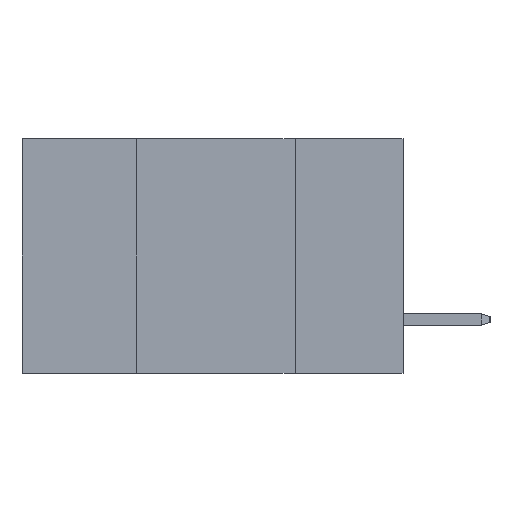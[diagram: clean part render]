
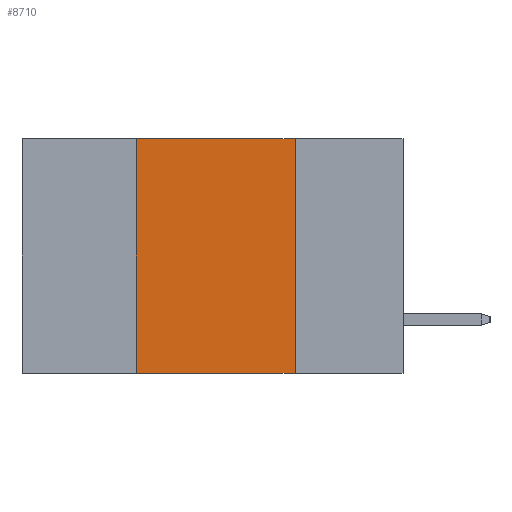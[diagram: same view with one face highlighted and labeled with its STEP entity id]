
A CAD part, left-side view. The second image highlights one B-rep face of the part: STEP entity #8710.
In plain terms, the highlighted planar face has unit normal (-1, 0, 0).
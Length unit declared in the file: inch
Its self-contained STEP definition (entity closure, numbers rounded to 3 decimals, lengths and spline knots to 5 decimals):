
#149 = CARTESIAN_POINT ( 'NONE',  ( 0., 0.6, 0. ) ) ;
#259 = CARTESIAN_POINT ( 'NONE',  ( 0., 0.6, -0.37 ) ) ;
#408 = EDGE_CURVE ( 'NONE', #11132, #8319, #11571, .T. ) ;
#747 = DIRECTION ( 'NONE',  ( 0., -1., 0. ) ) ;
#798 = CARTESIAN_POINT ( 'NONE',  ( 0., 0.42, 0. ) ) ;
#871 = CARTESIAN_POINT ( 'NONE',  ( 0., 0.42, 0. ) ) ;
#2020 = DIRECTION ( 'NONE',  ( 0., 0., -1. ) ) ;
#2052 = DIRECTION ( 'NONE',  ( 0., 0., -1. ) ) ;
#2926 = CARTESIAN_POINT ( 'NONE',  ( 0., 0.17, -0.37 ) ) ;
#3277 = EDGE_LOOP ( 'NONE', ( #5813, #7336, #9105, #10205 ) ) ;
#3893 = LINE ( 'NONE', #259, #6085 ) ;
#4747 = FACE_OUTER_BOUND ( 'NONE', #3277, .T. ) ;
#5245 = VECTOR ( 'NONE', #747, 39.37008 ) ;
#5610 = CARTESIAN_POINT ( 'NONE',  ( 0., 0.17, 0. ) ) ;
#5813 = ORIENTED_EDGE ( 'NONE', *, *, #9576, .F. ) ;
#6085 = VECTOR ( 'NONE', #10546, 39.37008 ) ;
#7280 = VECTOR ( 'NONE', #2052, 39.37008 ) ;
#7332 = CARTESIAN_POINT ( 'NONE',  ( 0., 0.42, -0.37 ) ) ;
#7336 = ORIENTED_EDGE ( 'NONE', *, *, #408, .F. ) ;
#8319 = VERTEX_POINT ( 'NONE', #9037 ) ;
#8391 = LINE ( 'NONE', #5610, #7280 ) ;
#8603 = PLANE ( 'NONE',  #8829 ) ;
#8710 = ADVANCED_FACE ( 'NONE', ( #4747 ), #8603, .F. ) ;
#8829 = AXIS2_PLACEMENT_3D ( 'NONE', #149, #11296, #2020 ) ;
#9037 = CARTESIAN_POINT ( 'NONE',  ( 0., 0.17, 0. ) ) ;
#9105 = ORIENTED_EDGE ( 'NONE', *, *, #11438, .F. ) ;
#9576 = EDGE_CURVE ( 'NONE', #8319, #11983, #8391, .T. ) ;
#9698 = CARTESIAN_POINT ( 'NONE',  ( 0., 0.6, 0. ) ) ;
#9874 = VERTEX_POINT ( 'NONE', #7332 ) ;
#10132 = DIRECTION ( 'NONE',  ( 0., 0., 1. ) ) ;
#10205 = ORIENTED_EDGE ( 'NONE', *, *, #10398, .T. ) ;
#10398 = EDGE_CURVE ( 'NONE', #9874, #11983, #3893, .T. ) ;
#10546 = DIRECTION ( 'NONE',  ( 0., -1., 0. ) ) ;
#10855 = LINE ( 'NONE', #798, #11397 ) ;
#11132 = VERTEX_POINT ( 'NONE', #871 ) ;
#11296 = DIRECTION ( 'NONE',  ( 1., 0., 0. ) ) ;
#11397 = VECTOR ( 'NONE', #10132, 39.37008 ) ;
#11438 = EDGE_CURVE ( 'NONE', #9874, #11132, #10855, .T. ) ;
#11571 = LINE ( 'NONE', #9698, #5245 ) ;
#11983 = VERTEX_POINT ( 'NONE', #2926 ) ;
